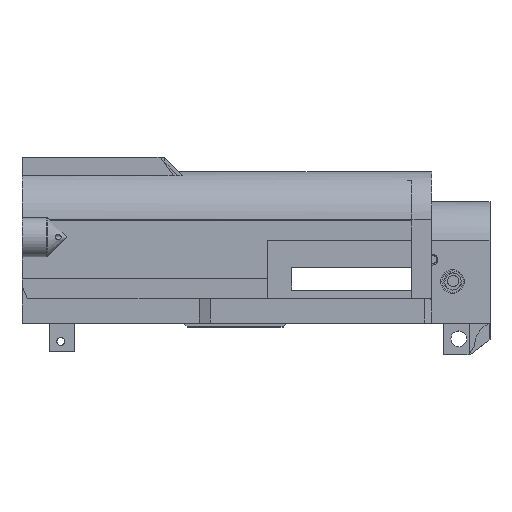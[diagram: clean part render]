
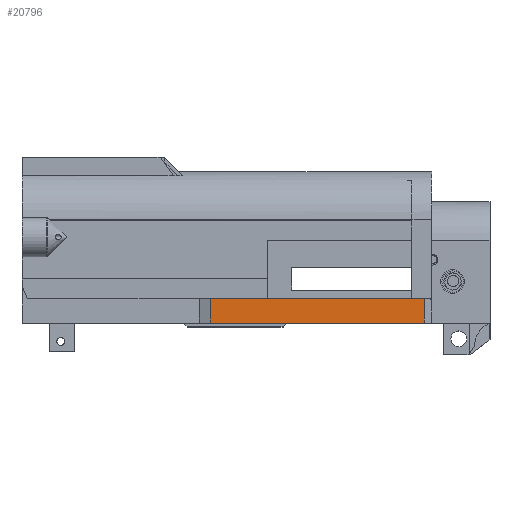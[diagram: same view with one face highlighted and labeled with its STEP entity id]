
A CAD part, top view. The second image highlights one B-rep face of the part: STEP entity #20796.
In plain terms, the highlighted planar face has unit normal (0, 0, 1).
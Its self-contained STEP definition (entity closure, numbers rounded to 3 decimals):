
#4663 = PLANE('',#4664);
#4664 = AXIS2_PLACEMENT_3D('',#4665,#4666,#4667);
#4665 = CARTESIAN_POINT('',(-105.565,16.363,18.567));
#4666 = DIRECTION('',(0.,1.,0.));
#4667 = DIRECTION('',(1.,0.,0.));
#11019 = PLANE('',#11020);
#11020 = AXIS2_PLACEMENT_3D('',#11021,#11022,#11023);
#11021 = CARTESIAN_POINT('',(-12.571,16.363,21.067));
#11022 = DIRECTION('',(0.707,0.,0.707));
#11023 = DIRECTION('',(0.,-1.,0.));
#12514 = EDGE_CURVE('',#12515,#12517,#12519,.T.);
#12515 = VERTEX_POINT('',#12516);
#12516 = CARTESIAN_POINT('',(-101.065,16.363,22.567));
#12517 = VERTEX_POINT('',#12518);
#12518 = CARTESIAN_POINT('',(-14.071,16.363,22.567));
#12519 = SURFACE_CURVE('',#12520,(#12524,#12531),.PCURVE_S1.);
#12520 = LINE('',#12521,#12522);
#12521 = CARTESIAN_POINT('',(-105.565,16.363,22.567));
#12522 = VECTOR('',#12523,1.);
#12523 = DIRECTION('',(1.,0.,0.));
#12524 = PCURVE('',#4663,#12525);
#12525 = DEFINITIONAL_REPRESENTATION('',(#12526),#12530);
#12526 = LINE('',#12527,#12528);
#12527 = CARTESIAN_POINT('',(0.,-4.));
#12528 = VECTOR('',#12529,1.);
#12529 = DIRECTION('',(1.,0.));
#12530 = ( GEOMETRIC_REPRESENTATION_CONTEXT(2) 
PARAMETRIC_REPRESENTATION_CONTEXT() REPRESENTATION_CONTEXT('2D SPACE',''
  ) );
#12531 = PCURVE('',#12532,#12537);
#12532 = PLANE('',#12533);
#12533 = AXIS2_PLACEMENT_3D('',#12534,#12535,#12536);
#12534 = CARTESIAN_POINT('',(-105.565,16.363,22.567));
#12535 = DIRECTION('',(0.,0.,1.));
#12536 = DIRECTION('',(1.,0.,0.));
#12537 = DEFINITIONAL_REPRESENTATION('',(#12538),#12542);
#12538 = LINE('',#12539,#12540);
#12539 = CARTESIAN_POINT('',(0.,0.));
#12540 = VECTOR('',#12541,1.);
#12541 = DIRECTION('',(1.,0.));
#12542 = ( GEOMETRIC_REPRESENTATION_CONTEXT(2) 
PARAMETRIC_REPRESENTATION_CONTEXT() REPRESENTATION_CONTEXT('2D SPACE',''
  ) );
#12677 = PLANE('',#12678);
#12678 = AXIS2_PLACEMENT_3D('',#12679,#12680,#12681);
#12679 = CARTESIAN_POINT('',(-103.199,6.363,21.683));
#12680 = DIRECTION('',(-0.383,0.,0.924));
#12681 = DIRECTION('',(0.,1.,0.));
#12775 = PLANE('',#12776);
#12776 = AXIS2_PLACEMENT_3D('',#12777,#12778,#12779);
#12777 = CARTESIAN_POINT('',(-11.071,6.363,18.567));
#12778 = DIRECTION('',(0.,-1.,0.));
#12779 = DIRECTION('',(-1.,0.,0.));
#18568 = EDGE_CURVE('',#12517,#18569,#18571,.T.);
#18569 = VERTEX_POINT('',#18570);
#18570 = CARTESIAN_POINT('',(-14.071,6.363,22.567));
#18571 = SURFACE_CURVE('',#18572,(#18576,#18583),.PCURVE_S1.);
#18572 = LINE('',#18573,#18574);
#18573 = CARTESIAN_POINT('',(-14.071,16.363,22.567));
#18574 = VECTOR('',#18575,1.);
#18575 = DIRECTION('',(0.,-1.,0.));
#18576 = PCURVE('',#11019,#18577);
#18577 = DEFINITIONAL_REPRESENTATION('',(#18578),#18582);
#18578 = LINE('',#18579,#18580);
#18579 = CARTESIAN_POINT('',(0.,-2.121));
#18580 = VECTOR('',#18581,1.);
#18581 = DIRECTION('',(1.,0.));
#18582 = ( GEOMETRIC_REPRESENTATION_CONTEXT(2) 
PARAMETRIC_REPRESENTATION_CONTEXT() REPRESENTATION_CONTEXT('2D SPACE',''
  ) );
#18583 = PCURVE('',#12532,#18584);
#18584 = DEFINITIONAL_REPRESENTATION('',(#18585),#18589);
#18585 = LINE('',#18586,#18587);
#18586 = CARTESIAN_POINT('',(91.494,0.));
#18587 = VECTOR('',#18588,1.);
#18588 = DIRECTION('',(0.,-1.));
#18589 = ( GEOMETRIC_REPRESENTATION_CONTEXT(2) 
PARAMETRIC_REPRESENTATION_CONTEXT() REPRESENTATION_CONTEXT('2D SPACE',''
  ) );
#20796 = ADVANCED_FACE('',(#20797),#12532,.T.);
#20797 = FACE_BOUND('',#20798,.T.);
#20798 = EDGE_LOOP('',(#20799,#20800,#20823,#20844));
#20799 = ORIENTED_EDGE('',*,*,#12514,.F.);
#20800 = ORIENTED_EDGE('',*,*,#20801,.F.);
#20801 = EDGE_CURVE('',#20802,#12515,#20804,.T.);
#20802 = VERTEX_POINT('',#20803);
#20803 = CARTESIAN_POINT('',(-101.065,6.363,22.567));
#20804 = SURFACE_CURVE('',#20805,(#20809,#20816),.PCURVE_S1.);
#20805 = LINE('',#20806,#20807);
#20806 = CARTESIAN_POINT('',(-101.065,6.363,22.567));
#20807 = VECTOR('',#20808,1.);
#20808 = DIRECTION('',(0.,1.,0.));
#20809 = PCURVE('',#12532,#20810);
#20810 = DEFINITIONAL_REPRESENTATION('',(#20811),#20815);
#20811 = LINE('',#20812,#20813);
#20812 = CARTESIAN_POINT('',(4.5,-10.));
#20813 = VECTOR('',#20814,1.);
#20814 = DIRECTION('',(0.,1.));
#20815 = ( GEOMETRIC_REPRESENTATION_CONTEXT(2) 
PARAMETRIC_REPRESENTATION_CONTEXT() REPRESENTATION_CONTEXT('2D SPACE',''
  ) );
#20816 = PCURVE('',#12677,#20817);
#20817 = DEFINITIONAL_REPRESENTATION('',(#20818),#20822);
#20818 = LINE('',#20819,#20820);
#20819 = CARTESIAN_POINT('',(0.,-2.31));
#20820 = VECTOR('',#20821,1.);
#20821 = DIRECTION('',(1.,0.));
#20822 = ( GEOMETRIC_REPRESENTATION_CONTEXT(2) 
PARAMETRIC_REPRESENTATION_CONTEXT() REPRESENTATION_CONTEXT('2D SPACE',''
  ) );
#20823 = ORIENTED_EDGE('',*,*,#20824,.F.);
#20824 = EDGE_CURVE('',#18569,#20802,#20825,.T.);
#20825 = SURFACE_CURVE('',#20826,(#20830,#20837),.PCURVE_S1.);
#20826 = LINE('',#20827,#20828);
#20827 = CARTESIAN_POINT('',(-11.071,6.363,22.567));
#20828 = VECTOR('',#20829,1.);
#20829 = DIRECTION('',(-1.,0.,0.));
#20830 = PCURVE('',#12532,#20831);
#20831 = DEFINITIONAL_REPRESENTATION('',(#20832),#20836);
#20832 = LINE('',#20833,#20834);
#20833 = CARTESIAN_POINT('',(94.494,-10.));
#20834 = VECTOR('',#20835,1.);
#20835 = DIRECTION('',(-1.,0.));
#20836 = ( GEOMETRIC_REPRESENTATION_CONTEXT(2) 
PARAMETRIC_REPRESENTATION_CONTEXT() REPRESENTATION_CONTEXT('2D SPACE',''
  ) );
#20837 = PCURVE('',#12775,#20838);
#20838 = DEFINITIONAL_REPRESENTATION('',(#20839),#20843);
#20839 = LINE('',#20840,#20841);
#20840 = CARTESIAN_POINT('',(0.,-4.));
#20841 = VECTOR('',#20842,1.);
#20842 = DIRECTION('',(1.,0.));
#20843 = ( GEOMETRIC_REPRESENTATION_CONTEXT(2) 
PARAMETRIC_REPRESENTATION_CONTEXT() REPRESENTATION_CONTEXT('2D SPACE',''
  ) );
#20844 = ORIENTED_EDGE('',*,*,#18568,.F.);
